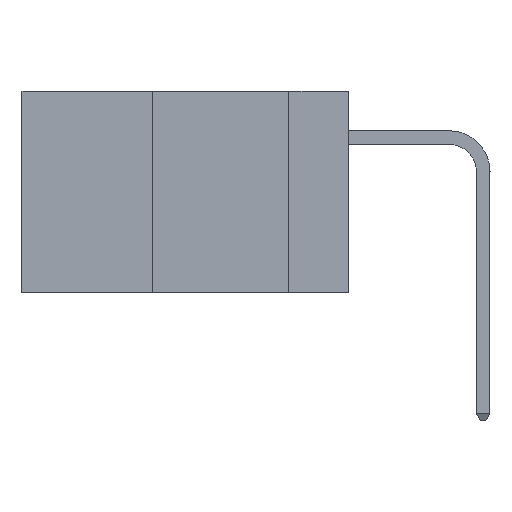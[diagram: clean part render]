
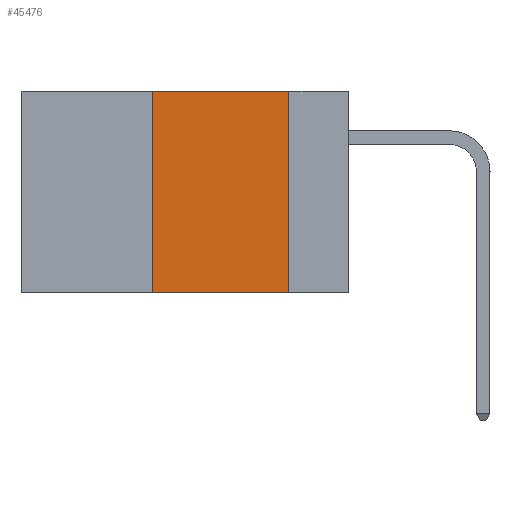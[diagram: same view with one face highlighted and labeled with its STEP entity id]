
A CAD part, left-side view. The second image highlights one B-rep face of the part: STEP entity #45476.
In plain terms, the highlighted planar face has unit normal (-1, 0, 0).
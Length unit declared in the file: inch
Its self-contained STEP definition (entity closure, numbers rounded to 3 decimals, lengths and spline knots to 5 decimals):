
#90 = DIRECTION ( 'NONE',  ( 0., -1., 0. ) ) ;
#520 = VERTEX_POINT ( 'NONE', #32571 ) ;
#3019 = LINE ( 'NONE', #34783, #32860 ) ;
#3276 = EDGE_CURVE ( 'NONE', #21026, #32359, #32323, .T. ) ;
#3882 = EDGE_CURVE ( 'NONE', #32359, #520, #3019, .T. ) ;
#4485 = VERTEX_POINT ( 'NONE', #26874 ) ;
#5234 = CARTESIAN_POINT ( 'NONE',  ( 0., 0.11, 0. ) ) ;
#6805 = CARTESIAN_POINT ( 'NONE',  ( 0., 0.6, 0. ) ) ;
#6993 = ORIENTED_EDGE ( 'NONE', *, *, #3882, .F. ) ;
#7255 = LINE ( 'NONE', #5234, #47392 ) ;
#10038 = EDGE_CURVE ( 'NONE', #520, #4485, #7255, .T. ) ;
#10646 = DIRECTION ( 'NONE',  ( 0., 0., -1. ) ) ;
#11815 = ORIENTED_EDGE ( 'NONE', *, *, #3276, .F. ) ;
#12988 = DIRECTION ( 'NONE',  ( 0., 0., -1. ) ) ;
#17026 = EDGE_LOOP ( 'NONE', ( #23998, #6993, #11815, #24044 ) ) ;
#18374 = LINE ( 'NONE', #45608, #39094 ) ;
#18384 = DIRECTION ( 'NONE',  ( 0., -1., 0. ) ) ;
#19636 = DIRECTION ( 'NONE',  ( 0., 0., 1. ) ) ;
#21026 = VERTEX_POINT ( 'NONE', #46850 ) ;
#21479 = EDGE_CURVE ( 'NONE', #21026, #4485, #18374, .T. ) ;
#23998 = ORIENTED_EDGE ( 'NONE', *, *, #10038, .F. ) ;
#24044 = ORIENTED_EDGE ( 'NONE', *, *, #21479, .T. ) ;
#26874 = CARTESIAN_POINT ( 'NONE',  ( 0., 0.11, -0.37 ) ) ;
#31871 = CARTESIAN_POINT ( 'NONE',  ( 0., 0.36, 0. ) ) ;
#32323 = LINE ( 'NONE', #35160, #42651 ) ;
#32359 = VERTEX_POINT ( 'NONE', #31871 ) ;
#32571 = CARTESIAN_POINT ( 'NONE',  ( 0., 0.11, 0. ) ) ;
#32860 = VECTOR ( 'NONE', #90, 39.37008 ) ;
#34044 = DIRECTION ( 'NONE',  ( 1., 0., 0. ) ) ;
#34783 = CARTESIAN_POINT ( 'NONE',  ( 0., 0.6, 0. ) ) ;
#35160 = CARTESIAN_POINT ( 'NONE',  ( 0., 0.36, 0. ) ) ;
#39094 = VECTOR ( 'NONE', #18384, 39.37008 ) ;
#42651 = VECTOR ( 'NONE', #19636, 39.37008 ) ;
#42724 = AXIS2_PLACEMENT_3D ( 'NONE', #6805, #34044, #10646 ) ;
#45476 = ADVANCED_FACE ( 'NONE', ( #47326 ), #45550, .F. ) ;
#45550 = PLANE ( 'NONE',  #42724 ) ;
#45608 = CARTESIAN_POINT ( 'NONE',  ( 0., 0.6, -0.37 ) ) ;
#46850 = CARTESIAN_POINT ( 'NONE',  ( 0., 0.36, -0.37 ) ) ;
#47326 = FACE_OUTER_BOUND ( 'NONE', #17026, .T. ) ;
#47392 = VECTOR ( 'NONE', #12988, 39.37008 ) ;
